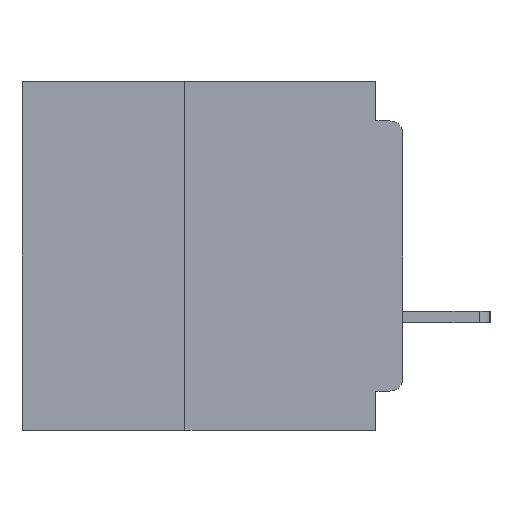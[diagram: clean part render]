
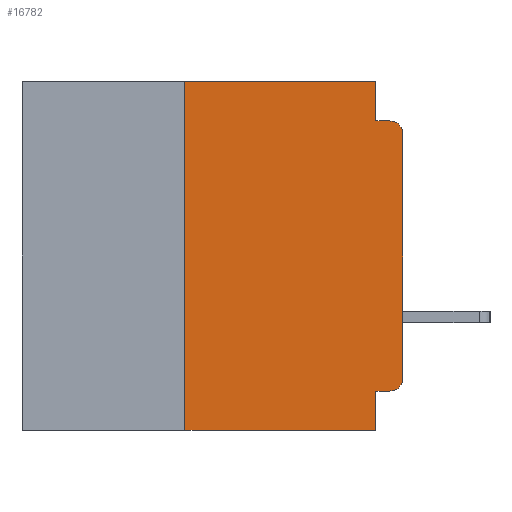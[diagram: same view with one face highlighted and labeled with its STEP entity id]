
A CAD part, left-side view. The second image highlights one B-rep face of the part: STEP entity #16782.
In plain terms, the highlighted planar face has unit normal (-1, 0, 0).
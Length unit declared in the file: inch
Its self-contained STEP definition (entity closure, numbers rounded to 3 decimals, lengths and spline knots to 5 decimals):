
#608 = EDGE_CURVE ( 'NONE', #38822, #3457, #23894, .T. ) ;
#1997 = CARTESIAN_POINT ( 'NONE',  ( 0., 0.031, 0. ) ) ;
#2556 = VECTOR ( 'NONE', #26031, 39.37008 ) ;
#2891 = AXIS2_PLACEMENT_3D ( 'NONE', #11199, #4004, #29214 ) ;
#3132 = LINE ( 'NONE', #10570, #22362 ) ;
#3457 = VERTEX_POINT ( 'NONE', #39040 ) ;
#3979 = LINE ( 'NONE', #5395, #39829 ) ;
#4004 = DIRECTION ( 'NONE',  ( 1., 0., 0. ) ) ;
#4648 = VERTEX_POINT ( 'NONE', #30900 ) ;
#4744 = AXIS2_PLACEMENT_3D ( 'NONE', #34188, #34097, #33890 ) ;
#4891 = CARTESIAN_POINT ( 'NONE',  ( 0., 0.015, -0.355 ) ) ;
#5395 = CARTESIAN_POINT ( 'NONE',  ( 0., 0.031, 0. ) ) ;
#6512 = EDGE_CURVE ( 'NONE', #33470, #7011, #16894, .T. ) ;
#7011 = VERTEX_POINT ( 'NONE', #15782 ) ;
#7593 = ORIENTED_EDGE ( 'NONE', *, *, #38499, .T. ) ;
#8185 = EDGE_CURVE ( 'NONE', #36594, #7011, #9405, .T. ) ;
#8512 = EDGE_CURVE ( 'NONE', #4648, #20392, #22269, .T. ) ;
#8699 = ORIENTED_EDGE ( 'NONE', *, *, #30754, .F. ) ;
#8911 = CIRCLE ( 'NONE', #9702, 0.015 ) ;
#9405 = LINE ( 'NONE', #44770, #46104 ) ;
#9702 = AXIS2_PLACEMENT_3D ( 'NONE', #42069, #20775, #45576 ) ;
#10570 = CARTESIAN_POINT ( 'NONE',  ( 0., 0.031, -0.4 ) ) ;
#10649 = EDGE_CURVE ( 'NONE', #23187, #36594, #3979, .T. ) ;
#11055 = LINE ( 'NONE', #17991, #38382 ) ;
#11199 = CARTESIAN_POINT ( 'NONE',  ( 0., 0.437, 0. ) ) ;
#11746 = CARTESIAN_POINT ( 'NONE',  ( 0., 0.25, -0.4 ) ) ;
#12079 = ORIENTED_EDGE ( 'NONE', *, *, #32935, .T. ) ;
#12119 = ORIENTED_EDGE ( 'NONE', *, *, #26393, .F. ) ;
#12763 = VECTOR ( 'NONE', #38955, 39.37008 ) ;
#14750 = CARTESIAN_POINT ( 'NONE',  ( 0., 0., -0.06 ) ) ;
#15263 = CARTESIAN_POINT ( 'NONE',  ( 0., 0., 0. ) ) ;
#15782 = CARTESIAN_POINT ( 'NONE',  ( 0., 0.015, -0.045 ) ) ;
#16578 = ORIENTED_EDGE ( 'NONE', *, *, #6512, .T. ) ;
#16782 = ADVANCED_FACE ( 'NONE', ( #28951 ), #18396, .F. ) ;
#16894 = CIRCLE ( 'NONE', #4744, 0.015 ) ;
#16942 = CARTESIAN_POINT ( 'NONE',  ( 0., 0.031, -0.4 ) ) ;
#17991 = CARTESIAN_POINT ( 'NONE',  ( 0., 0.437, 0. ) ) ;
#18396 = PLANE ( 'NONE',  #2891 ) ;
#20204 = VERTEX_POINT ( 'NONE', #33659 ) ;
#20392 = VERTEX_POINT ( 'NONE', #16942 ) ;
#20775 = DIRECTION ( 'NONE',  ( -1., 0., 0. ) ) ;
#21054 = ORIENTED_EDGE ( 'NONE', *, *, #608, .F. ) ;
#22123 = EDGE_CURVE ( 'NONE', #3457, #20392, #3132, .T. ) ;
#22269 = LINE ( 'NONE', #38994, #12763 ) ;
#22362 = VECTOR ( 'NONE', #46137, 39.37008 ) ;
#23187 = VERTEX_POINT ( 'NONE', #1997 ) ;
#23894 = LINE ( 'NONE', #41343, #38324 ) ;
#25016 = ORIENTED_EDGE ( 'NONE', *, *, #8512, .T. ) ;
#26031 = DIRECTION ( 'NONE',  ( 0., 0., 1. ) ) ;
#26091 = DIRECTION ( 'NONE',  ( 0., 0., 1. ) ) ;
#26393 = EDGE_CURVE ( 'NONE', #4648, #45545, #41161, .T. ) ;
#26542 = VECTOR ( 'NONE', #26091, 39.37008 ) ;
#26686 = ORIENTED_EDGE ( 'NONE', *, *, #10649, .F. ) ;
#26996 = DIRECTION ( 'NONE',  ( 0., 0., -1. ) ) ;
#28058 = EDGE_LOOP ( 'NONE', ( #12079, #16578, #38826, #26686, #8699, #12119, #25016, #37786, #21054, #7593 ) ) ;
#28793 = DIRECTION ( 'NONE',  ( 0., -1., 0. ) ) ;
#28951 = FACE_OUTER_BOUND ( 'NONE', #28058, .T. ) ;
#29214 = DIRECTION ( 'NONE',  ( 0., 0., -1. ) ) ;
#30754 = EDGE_CURVE ( 'NONE', #45545, #23187, #11055, .T. ) ;
#30900 = CARTESIAN_POINT ( 'NONE',  ( 0., 0.25, -0.4 ) ) ;
#32935 = EDGE_CURVE ( 'NONE', #20204, #33470, #45306, .T. ) ;
#33470 = VERTEX_POINT ( 'NONE', #14750 ) ;
#33659 = CARTESIAN_POINT ( 'NONE',  ( 0., 0., -0.34 ) ) ;
#33890 = DIRECTION ( 'NONE',  ( 0., 0., -1. ) ) ;
#34097 = DIRECTION ( 'NONE',  ( -1., 0., 0. ) ) ;
#34188 = CARTESIAN_POINT ( 'NONE',  ( 0., 0.015, -0.06 ) ) ;
#34550 = CARTESIAN_POINT ( 'NONE',  ( 0., 0.25, 0. ) ) ;
#36594 = VERTEX_POINT ( 'NONE', #44678 ) ;
#37786 = ORIENTED_EDGE ( 'NONE', *, *, #22123, .F. ) ;
#38115 = DIRECTION ( 'NONE',  ( 0., 1., 0. ) ) ;
#38324 = VECTOR ( 'NONE', #38115, 39.37008 ) ;
#38382 = VECTOR ( 'NONE', #28793, 39.37008 ) ;
#38499 = EDGE_CURVE ( 'NONE', #38822, #20204, #8911, .T. ) ;
#38822 = VERTEX_POINT ( 'NONE', #4891 ) ;
#38826 = ORIENTED_EDGE ( 'NONE', *, *, #8185, .F. ) ;
#38955 = DIRECTION ( 'NONE',  ( 0., -1., 0. ) ) ;
#38994 = CARTESIAN_POINT ( 'NONE',  ( 0., 0.437, -0.4 ) ) ;
#39040 = CARTESIAN_POINT ( 'NONE',  ( 0., 0.031, -0.355 ) ) ;
#39829 = VECTOR ( 'NONE', #26996, 39.37008 ) ;
#41161 = LINE ( 'NONE', #11746, #2556 ) ;
#41343 = CARTESIAN_POINT ( 'NONE',  ( 0., 0., -0.355 ) ) ;
#42069 = CARTESIAN_POINT ( 'NONE',  ( 0., 0.015, -0.34 ) ) ;
#44678 = CARTESIAN_POINT ( 'NONE',  ( 0., 0.031, -0.045 ) ) ;
#44711 = DIRECTION ( 'NONE',  ( 0., -1., 0. ) ) ;
#44770 = CARTESIAN_POINT ( 'NONE',  ( 0., 0., -0.045 ) ) ;
#45306 = LINE ( 'NONE', #15263, #26542 ) ;
#45545 = VERTEX_POINT ( 'NONE', #34550 ) ;
#45576 = DIRECTION ( 'NONE',  ( 0., 0., -1. ) ) ;
#46104 = VECTOR ( 'NONE', #44711, 39.37008 ) ;
#46137 = DIRECTION ( 'NONE',  ( 0., 0., -1. ) ) ;
